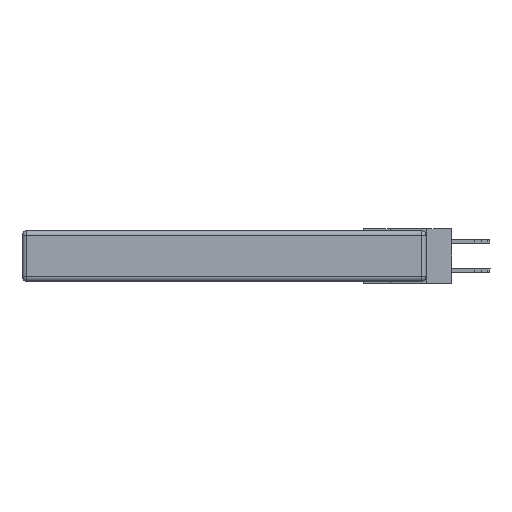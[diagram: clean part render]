
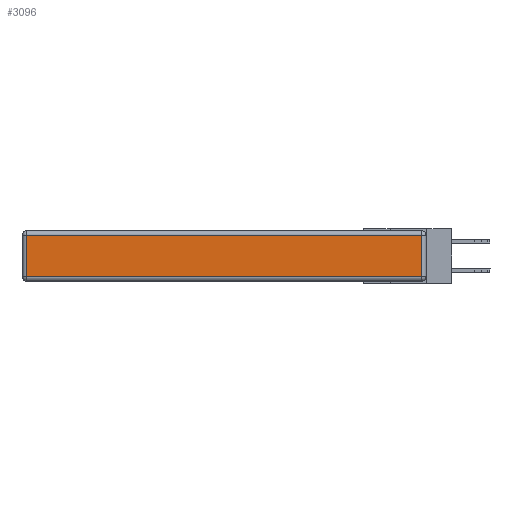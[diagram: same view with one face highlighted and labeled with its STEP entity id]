
A CAD part, left-side view. The second image highlights one B-rep face of the part: STEP entity #3096.
In plain terms, the highlighted planar face has unit normal (-1, 0, 0).
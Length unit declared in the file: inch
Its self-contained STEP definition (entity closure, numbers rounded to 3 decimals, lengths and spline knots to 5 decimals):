
#816 = ORIENTED_EDGE ( 'NONE', *, *, #11485, .T. ) ;
#990 = DIRECTION ( 'NONE',  ( 0., 0., -1. ) ) ;
#1993 = EDGE_CURVE ( 'NONE', #22292, #22096, #15488, .T. ) ;
#2182 = CARTESIAN_POINT ( 'NONE',  ( 0., 2.72, -0.313 ) ) ;
#2465 = VERTEX_POINT ( 'NONE', #4558 ) ;
#2673 = CARTESIAN_POINT ( 'NONE',  ( 0., 2.72, -0.343 ) ) ;
#3059 = VECTOR ( 'NONE', #6514, 39.37008 ) ;
#3096 = ADVANCED_FACE ( 'NONE', ( #14533 ), #5658, .T. ) ;
#3872 = VERTEX_POINT ( 'NONE', #8632 ) ;
#4558 = CARTESIAN_POINT ( 'NONE',  ( 0., 0.03, -0.313 ) ) ;
#4787 = CARTESIAN_POINT ( 'NONE',  ( 0., 2.72, -0.03 ) ) ;
#5658 = PLANE ( 'NONE',  #16910 ) ;
#6514 = DIRECTION ( 'NONE',  ( 0., 0., 1. ) ) ;
#8512 = DIRECTION ( 'NONE',  ( 0., 1., 0. ) ) ;
#8632 = CARTESIAN_POINT ( 'NONE',  ( 0., 0.03, -0.03 ) ) ;
#8769 = VECTOR ( 'NONE', #8512, 39.37008 ) ;
#11378 = CARTESIAN_POINT ( 'NONE',  ( 0., 0.03, -0.343 ) ) ;
#11485 = EDGE_CURVE ( 'NONE', #2465, #3872, #24524, .T. ) ;
#14533 = FACE_OUTER_BOUND ( 'NONE', #14984, .T. ) ;
#14984 = EDGE_LOOP ( 'NONE', ( #17823, #816, #22156, #26379 ) ) ;
#15038 = LINE ( 'NONE', #23700, #27164 ) ;
#15488 = LINE ( 'NONE', #2673, #28279 ) ;
#16910 = AXIS2_PLACEMENT_3D ( 'NONE', #28640, #28431, #19248 ) ;
#17156 = CARTESIAN_POINT ( 'NONE',  ( 0., 2.75, -0.03 ) ) ;
#17823 = ORIENTED_EDGE ( 'NONE', *, *, #23840, .T. ) ;
#19248 = DIRECTION ( 'NONE',  ( 0., 0., 1. ) ) ;
#19492 = DIRECTION ( 'NONE',  ( 0., -1., 0. ) ) ;
#20901 = LINE ( 'NONE', #17156, #8769 ) ;
#21020 = EDGE_CURVE ( 'NONE', #3872, #22292, #20901, .T. ) ;
#22096 = VERTEX_POINT ( 'NONE', #2182 ) ;
#22156 = ORIENTED_EDGE ( 'NONE', *, *, #21020, .T. ) ;
#22292 = VERTEX_POINT ( 'NONE', #4787 ) ;
#23700 = CARTESIAN_POINT ( 'NONE',  ( 0., 0., -0.313 ) ) ;
#23840 = EDGE_CURVE ( 'NONE', #22096, #2465, #15038, .T. ) ;
#24524 = LINE ( 'NONE', #11378, #3059 ) ;
#26379 = ORIENTED_EDGE ( 'NONE', *, *, #1993, .T. ) ;
#27164 = VECTOR ( 'NONE', #19492, 39.37008 ) ;
#28279 = VECTOR ( 'NONE', #990, 39.37008 ) ;
#28431 = DIRECTION ( 'NONE',  ( -1., 0., 0. ) ) ;
#28640 = CARTESIAN_POINT ( 'NONE',  ( 0., 0., -0.343 ) ) ;
